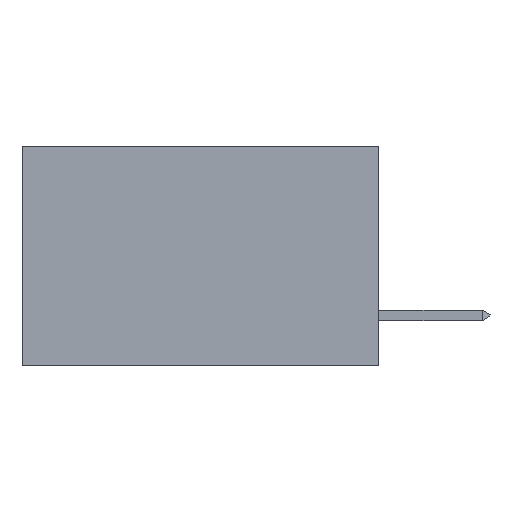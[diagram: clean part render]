
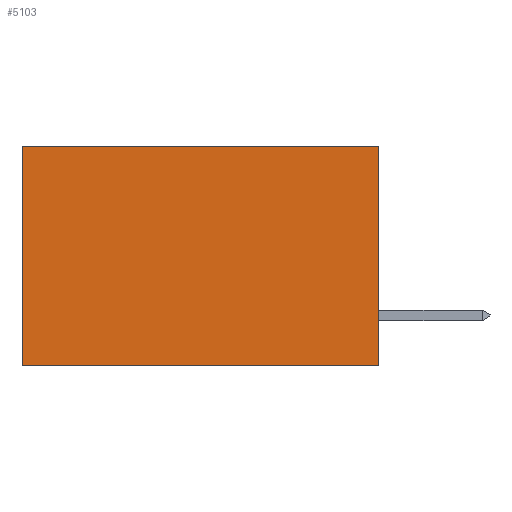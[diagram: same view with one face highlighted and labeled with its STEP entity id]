
A CAD part, left-side view. The second image highlights one B-rep face of the part: STEP entity #5103.
In plain terms, the highlighted planar face has unit normal (-1, 0, 0).
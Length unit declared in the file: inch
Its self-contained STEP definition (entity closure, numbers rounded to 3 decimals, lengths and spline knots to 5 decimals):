
#316 = EDGE_CURVE ( 'NONE', #920, #20227, #21009, .T. ) ;
#359 = DIRECTION ( 'NONE',  ( 1., 0., 0. ) ) ;
#431 = ORIENTED_EDGE ( 'NONE', *, *, #6513, .F. ) ;
#870 = CARTESIAN_POINT ( 'NONE',  ( 0.298, 0., 0. ) ) ;
#920 = VERTEX_POINT ( 'NONE', #3176 ) ;
#1953 = VERTEX_POINT ( 'NONE', #29226 ) ;
#2314 = PLANE ( 'NONE',  #20481 ) ;
#2938 = EDGE_CURVE ( 'NONE', #15567, #20227, #22570, .T. ) ;
#3176 = CARTESIAN_POINT ( 'NONE',  ( 0.298, 0.6, 0. ) ) ;
#4516 = DIRECTION ( 'NONE',  ( 0., 0., -1. ) ) ;
#4736 = CARTESIAN_POINT ( 'NONE',  ( 0.298, 0., 0. ) ) ;
#5103 = ADVANCED_FACE ( 'NONE', ( #10723 ), #2314, .F. ) ;
#6513 = EDGE_CURVE ( 'NONE', #1953, #15567, #28970, .T. ) ;
#7035 = VECTOR ( 'NONE', #23556, 39.37008 ) ;
#7060 = DIRECTION ( 'NONE',  ( 0., 1., 0. ) ) ;
#8744 = ORIENTED_EDGE ( 'NONE', *, *, #2938, .F. ) ;
#9100 = CARTESIAN_POINT ( 'NONE',  ( 0.298, 0.6, 0. ) ) ;
#9165 = CARTESIAN_POINT ( 'NONE',  ( 0.298, 0., 0. ) ) ;
#9265 = ORIENTED_EDGE ( 'NONE', *, *, #316, .T. ) ;
#10723 = FACE_OUTER_BOUND ( 'NONE', #25962, .T. ) ;
#11168 = DIRECTION ( 'NONE',  ( 0., 0., -1. ) ) ;
#14754 = LINE ( 'NONE', #870, #7035 ) ;
#15567 = VERTEX_POINT ( 'NONE', #20687 ) ;
#16168 = CARTESIAN_POINT ( 'NONE',  ( 0.298, 0., -0.37 ) ) ;
#16227 = DIRECTION ( 'NONE',  ( 0., 0., -1. ) ) ;
#16456 = EDGE_CURVE ( 'NONE', #1953, #920, #14754, .T. ) ;
#20223 = ORIENTED_EDGE ( 'NONE', *, *, #16456, .T. ) ;
#20227 = VERTEX_POINT ( 'NONE', #23756 ) ;
#20481 = AXIS2_PLACEMENT_3D ( 'NONE', #9165, #359, #4516 ) ;
#20687 = CARTESIAN_POINT ( 'NONE',  ( 0.298, 0., -0.37 ) ) ;
#21009 = LINE ( 'NONE', #9100, #28729 ) ;
#22570 = LINE ( 'NONE', #16168, #26101 ) ;
#23556 = DIRECTION ( 'NONE',  ( 0., 1., 0. ) ) ;
#23756 = CARTESIAN_POINT ( 'NONE',  ( 0.298, 0.6, -0.37 ) ) ;
#25962 = EDGE_LOOP ( 'NONE', ( #9265, #8744, #431, #20223 ) ) ;
#26101 = VECTOR ( 'NONE', #7060, 39.37008 ) ;
#27567 = VECTOR ( 'NONE', #16227, 39.37008 ) ;
#28729 = VECTOR ( 'NONE', #11168, 39.37008 ) ;
#28970 = LINE ( 'NONE', #4736, #27567 ) ;
#29226 = CARTESIAN_POINT ( 'NONE',  ( 0.298, 0., 0. ) ) ;
